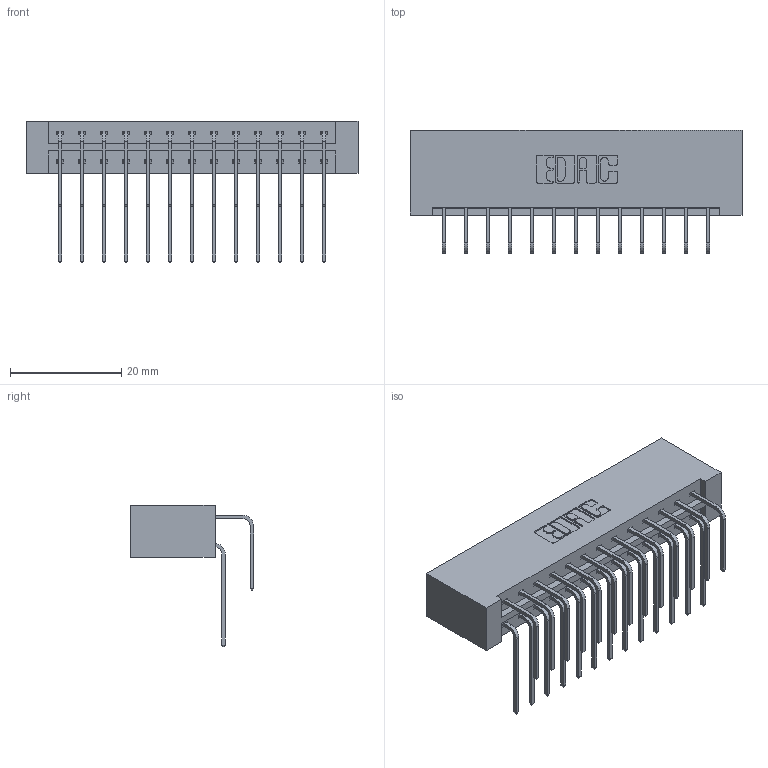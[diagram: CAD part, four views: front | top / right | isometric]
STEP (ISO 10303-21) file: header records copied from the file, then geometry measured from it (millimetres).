
FILE_DESCRIPTION (( 'STEP AP203' ), '1' );
FILE_NAME ('333-026-558-201.STEP', '2018-08-02T13:23:34', ( '' ), ( '' ), 'SwSTEP 2.0', 'SolidWorks 2016', '' );
FILE_SCHEMA (( 'CONFIG_CONTROL_DESIGN' ));
Length unit declared in the file: inch
Products named in the file (4): 333 Part_Lugless; 345-292-001_558 559 Tail - 1; 345-292-001_558 Tail - 2; 333-026-558-201
Assembly tree (27 placements, depth 2):
  333-026-558-201
    333 Part_Lugless
    345-292-001_558 559 Tail - 1  x13
    345-292-001_558 Tail - 2  x13
Bounding box: 59.77 x 22.17 x 25.53 mm (x, y, z)
Volume: 6612.8 mm3; surface area: 8277.8 mm2
Topology: 27 solids, 27 shells, 1510 faces, 4473 edges, 2946 vertices
Faces by surface type: plane 1054, cylinder 456
Entity records: 13621 total; most frequent: CARTESIAN_POINT 2341, ORIENTED_EDGE 2226, DIRECTION 2025, EDGE_CURVE 1113, LINE 953, VECTOR 953, VERTEX_POINT 738, AXIS2_PLACEMENT_3D 536
